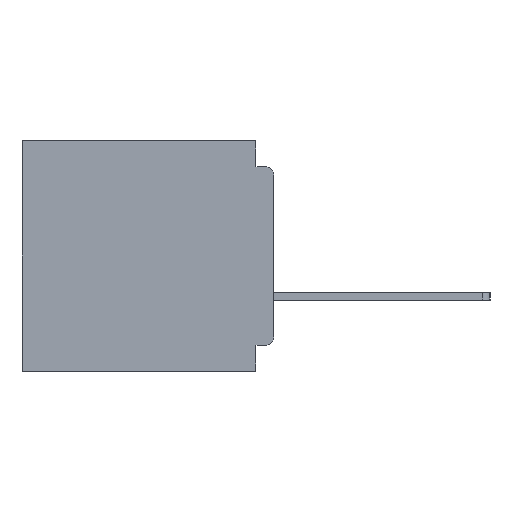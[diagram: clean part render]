
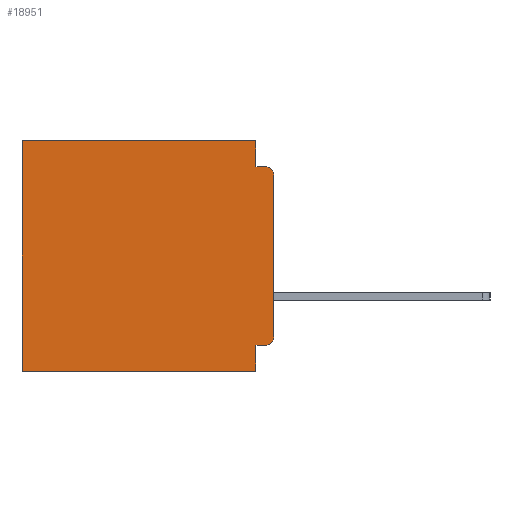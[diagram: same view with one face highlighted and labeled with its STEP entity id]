
A CAD part, left-side view. The second image highlights one B-rep face of the part: STEP entity #18951.
In plain terms, the highlighted planar face has unit normal (-1, 0, 0).
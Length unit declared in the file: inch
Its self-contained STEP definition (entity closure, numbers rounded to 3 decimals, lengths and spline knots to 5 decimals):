
#688 = ORIENTED_EDGE ( 'NONE', *, *, #41181, .F. ) ;
#1342 = DIRECTION ( 'NONE',  ( 0., 1., 0. ) ) ;
#1982 = DIRECTION ( 'NONE',  ( 0., 0., -1. ) ) ;
#2154 = CARTESIAN_POINT ( 'NONE',  ( 0.3, 0.437, -0.4 ) ) ;
#2302 = DIRECTION ( 'NONE',  ( 0., 0., -1. ) ) ;
#2315 = LINE ( 'NONE', #15411, #10452 ) ;
#2664 = CARTESIAN_POINT ( 'NONE',  ( 0.3, 0., -0.4 ) ) ;
#3512 = CARTESIAN_POINT ( 'NONE',  ( 0.3, 0.031, 0. ) ) ;
#3690 = CARTESIAN_POINT ( 'NONE',  ( 0.3, 0.437, 0. ) ) ;
#4051 = EDGE_CURVE ( 'NONE', #30964, #38683, #34773, .T. ) ;
#5552 = VERTEX_POINT ( 'NONE', #33634 ) ;
#6205 = DIRECTION ( 'NONE',  ( 0., 1., 0. ) ) ;
#7427 = ORIENTED_EDGE ( 'NONE', *, *, #31889, .T. ) ;
#7983 = EDGE_LOOP ( 'NONE', ( #28055, #25496, #14577, #688, #15071, #7427, #15714, #28582, #43833, #20281 ) ) ;
#8104 = AXIS2_PLACEMENT_3D ( 'NONE', #9639, #33281, #13038 ) ;
#8486 = CARTESIAN_POINT ( 'NONE',  ( 0.3, 0., -0.4 ) ) ;
#9639 = CARTESIAN_POINT ( 'NONE',  ( 0.3, 0.015, -0.06 ) ) ;
#10044 = CARTESIAN_POINT ( 'NONE',  ( 0.3, 0.031, -0.4 ) ) ;
#10452 = VECTOR ( 'NONE', #18677, 39.37008 ) ;
#10733 = VECTOR ( 'NONE', #1982, 39.37008 ) ;
#10942 = CARTESIAN_POINT ( 'NONE',  ( 0.3, 0., -0.34 ) ) ;
#11793 = LINE ( 'NONE', #39390, #10733 ) ;
#11902 = LINE ( 'NONE', #25167, #38858 ) ;
#12182 = VERTEX_POINT ( 'NONE', #37432 ) ;
#13038 = DIRECTION ( 'NONE',  ( 0., 0., -1. ) ) ;
#14344 = CARTESIAN_POINT ( 'NONE',  ( 0.3, 0.031, -0.4 ) ) ;
#14577 = ORIENTED_EDGE ( 'NONE', *, *, #36548, .F. ) ;
#14601 = VERTEX_POINT ( 'NONE', #3690 ) ;
#14719 = CARTESIAN_POINT ( 'NONE',  ( 0.3, 0.015, -0.34 ) ) ;
#14942 = EDGE_CURVE ( 'NONE', #26234, #40398, #11793, .T. ) ;
#15071 = ORIENTED_EDGE ( 'NONE', *, *, #42587, .T. ) ;
#15411 = CARTESIAN_POINT ( 'NONE',  ( 0.3, 0.031, 0. ) ) ;
#15714 = ORIENTED_EDGE ( 'NONE', *, *, #24936, .F. ) ;
#16827 = VECTOR ( 'NONE', #27098, 39.37008 ) ;
#17006 = AXIS2_PLACEMENT_3D ( 'NONE', #14719, #38415, #18135 ) ;
#17645 = LINE ( 'NONE', #2664, #34639 ) ;
#18135 = DIRECTION ( 'NONE',  ( 0., 0., -1. ) ) ;
#18647 = DIRECTION ( 'NONE',  ( 0., 0., -1. ) ) ;
#18677 = DIRECTION ( 'NONE',  ( 0., 0., -1. ) ) ;
#18951 = ADVANCED_FACE ( 'NONE', ( #43872 ), #42017, .F. ) ;
#20281 = ORIENTED_EDGE ( 'NONE', *, *, #31751, .T. ) ;
#21841 = DIRECTION ( 'NONE',  ( 0., -1., 0. ) ) ;
#21988 = AXIS2_PLACEMENT_3D ( 'NONE', #8486, #38929, #18647 ) ;
#22393 = EDGE_CURVE ( 'NONE', #31669, #30964, #43735, .T. ) ;
#22697 = CIRCLE ( 'NONE', #17006, 0.015 ) ;
#23661 = CARTESIAN_POINT ( 'NONE',  ( 0.3, 0., -0.355 ) ) ;
#23828 = LINE ( 'NONE', #38732, #31799 ) ;
#24936 = EDGE_CURVE ( 'NONE', #38683, #27208, #17645, .T. ) ;
#25167 = CARTESIAN_POINT ( 'NONE',  ( 0.3, 0., 0. ) ) ;
#25496 = ORIENTED_EDGE ( 'NONE', *, *, #36178, .T. ) ;
#26171 = DIRECTION ( 'NONE',  ( 0., 0., -1. ) ) ;
#26234 = VERTEX_POINT ( 'NONE', #39967 ) ;
#27098 = DIRECTION ( 'NONE',  ( 0., 1., 0. ) ) ;
#27208 = VERTEX_POINT ( 'NONE', #41656 ) ;
#28055 = ORIENTED_EDGE ( 'NONE', *, *, #14942, .F. ) ;
#28582 = ORIENTED_EDGE ( 'NONE', *, *, #4051, .F. ) ;
#30521 = CARTESIAN_POINT ( 'NONE',  ( 0.3, 0.031, -0.355 ) ) ;
#30964 = VERTEX_POINT ( 'NONE', #30521 ) ;
#31669 = VERTEX_POINT ( 'NONE', #37680 ) ;
#31751 = EDGE_CURVE ( 'NONE', #31669, #40398, #22697, .T. ) ;
#31799 = VECTOR ( 'NONE', #21841, 39.37008 ) ;
#31838 = CIRCLE ( 'NONE', #8104, 0.015 ) ;
#31889 = EDGE_CURVE ( 'NONE', #14601, #27208, #35455, .T. ) ;
#33281 = DIRECTION ( 'NONE',  ( -1., 0., 0. ) ) ;
#33634 = CARTESIAN_POINT ( 'NONE',  ( 0.3, 0.015, -0.045 ) ) ;
#33682 = VECTOR ( 'NONE', #26171, 39.37008 ) ;
#34407 = VECTOR ( 'NONE', #2302, 39.37008 ) ;
#34639 = VECTOR ( 'NONE', #6205, 39.37008 ) ;
#34773 = LINE ( 'NONE', #14344, #33682 ) ;
#35455 = LINE ( 'NONE', #2154, #34407 ) ;
#35743 = VERTEX_POINT ( 'NONE', #3512 ) ;
#36178 = EDGE_CURVE ( 'NONE', #26234, #5552, #31838, .T. ) ;
#36548 = EDGE_CURVE ( 'NONE', #12182, #5552, #23828, .T. ) ;
#37432 = CARTESIAN_POINT ( 'NONE',  ( 0.3, 0.031, -0.045 ) ) ;
#37680 = CARTESIAN_POINT ( 'NONE',  ( 0.3, 0.015, -0.355 ) ) ;
#38415 = DIRECTION ( 'NONE',  ( -1., 0., 0. ) ) ;
#38683 = VERTEX_POINT ( 'NONE', #10044 ) ;
#38732 = CARTESIAN_POINT ( 'NONE',  ( 0.3, 0., -0.045 ) ) ;
#38858 = VECTOR ( 'NONE', #1342, 39.37008 ) ;
#38929 = DIRECTION ( 'NONE',  ( 1., 0., 0. ) ) ;
#39390 = CARTESIAN_POINT ( 'NONE',  ( 0.3, 0., -0.4 ) ) ;
#39967 = CARTESIAN_POINT ( 'NONE',  ( 0.3, 0., -0.06 ) ) ;
#40398 = VERTEX_POINT ( 'NONE', #10942 ) ;
#41181 = EDGE_CURVE ( 'NONE', #35743, #12182, #2315, .T. ) ;
#41656 = CARTESIAN_POINT ( 'NONE',  ( 0.3, 0.437, -0.4 ) ) ;
#42017 = PLANE ( 'NONE',  #21988 ) ;
#42587 = EDGE_CURVE ( 'NONE', #35743, #14601, #11902, .T. ) ;
#43735 = LINE ( 'NONE', #23661, #16827 ) ;
#43833 = ORIENTED_EDGE ( 'NONE', *, *, #22393, .F. ) ;
#43872 = FACE_OUTER_BOUND ( 'NONE', #7983, .T. ) ;
